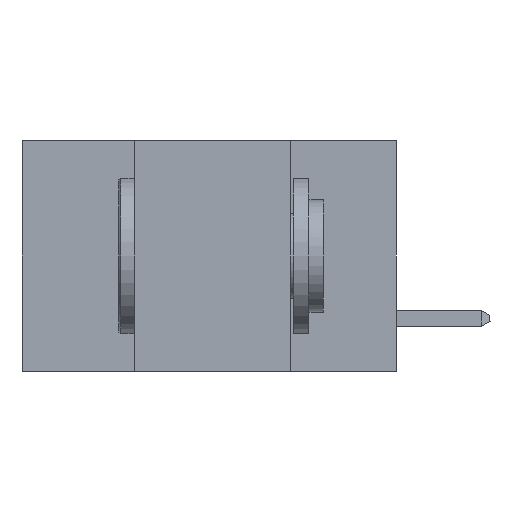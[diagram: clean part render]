
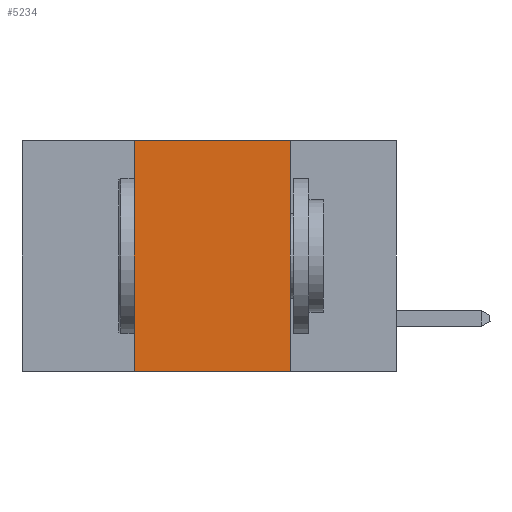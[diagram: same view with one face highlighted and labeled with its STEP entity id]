
A CAD part, left-side view. The second image highlights one B-rep face of the part: STEP entity #5234.
In plain terms, the highlighted planar face has unit normal (-1, 0, 0).
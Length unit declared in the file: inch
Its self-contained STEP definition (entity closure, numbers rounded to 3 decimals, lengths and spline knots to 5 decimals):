
#939 = DIRECTION ( 'NONE',  ( 0., 0., -1. ) ) ;
#1026 = CARTESIAN_POINT ( 'NONE',  ( 0., 0.42, 0. ) ) ;
#1321 = PLANE ( 'NONE',  #9477 ) ;
#1490 = ORIENTED_EDGE ( 'NONE', *, *, #14654, .F. ) ;
#1694 = DIRECTION ( 'NONE',  ( 0., -1., 0. ) ) ;
#2045 = EDGE_LOOP ( 'NONE', ( #12475, #1490, #8329, #12828 ) ) ;
#2489 = EDGE_CURVE ( 'NONE', #9586, #12381, #11811, .T. ) ;
#2988 = CARTESIAN_POINT ( 'NONE',  ( 0., 0.6, 0. ) ) ;
#3374 = VECTOR ( 'NONE', #4443, 39.37008 ) ;
#4443 = DIRECTION ( 'NONE',  ( 0., 0., 1. ) ) ;
#5234 = ADVANCED_FACE ( 'NONE', ( #7998 ), #1321, .F. ) ;
#5679 = VECTOR ( 'NONE', #13237, 39.37008 ) ;
#5770 = LINE ( 'NONE', #14671, #11549 ) ;
#6083 = VECTOR ( 'NONE', #1694, 39.37008 ) ;
#6696 = EDGE_CURVE ( 'NONE', #12241, #12381, #5770, .T. ) ;
#7849 = CARTESIAN_POINT ( 'NONE',  ( 0., 0.42, 0. ) ) ;
#7998 = FACE_OUTER_BOUND ( 'NONE', #2045, .T. ) ;
#8269 = CARTESIAN_POINT ( 'NONE',  ( 0., 0.17, -0.37 ) ) ;
#8329 = ORIENTED_EDGE ( 'NONE', *, *, #10564, .F. ) ;
#9477 = AXIS2_PLACEMENT_3D ( 'NONE', #2988, #11970, #11953 ) ;
#9543 = LINE ( 'NONE', #10909, #6083 ) ;
#9586 = VERTEX_POINT ( 'NONE', #13926 ) ;
#10326 = CARTESIAN_POINT ( 'NONE',  ( 0., 0.17, 0. ) ) ;
#10564 = EDGE_CURVE ( 'NONE', #9586, #13044, #12161, .T. ) ;
#10909 = CARTESIAN_POINT ( 'NONE',  ( 0., 0.6, 0. ) ) ;
#11549 = VECTOR ( 'NONE', #939, 39.37008 ) ;
#11811 = LINE ( 'NONE', #12761, #5679 ) ;
#11953 = DIRECTION ( 'NONE',  ( 0., 0., -1. ) ) ;
#11970 = DIRECTION ( 'NONE',  ( 1., 0., 0. ) ) ;
#12161 = LINE ( 'NONE', #1026, #3374 ) ;
#12241 = VERTEX_POINT ( 'NONE', #10326 ) ;
#12381 = VERTEX_POINT ( 'NONE', #8269 ) ;
#12475 = ORIENTED_EDGE ( 'NONE', *, *, #6696, .F. ) ;
#12761 = CARTESIAN_POINT ( 'NONE',  ( 0., 0.6, -0.37 ) ) ;
#12828 = ORIENTED_EDGE ( 'NONE', *, *, #2489, .T. ) ;
#13044 = VERTEX_POINT ( 'NONE', #7849 ) ;
#13237 = DIRECTION ( 'NONE',  ( 0., -1., 0. ) ) ;
#13926 = CARTESIAN_POINT ( 'NONE',  ( 0., 0.42, -0.37 ) ) ;
#14654 = EDGE_CURVE ( 'NONE', #13044, #12241, #9543, .T. ) ;
#14671 = CARTESIAN_POINT ( 'NONE',  ( 0., 0.17, 0. ) ) ;
